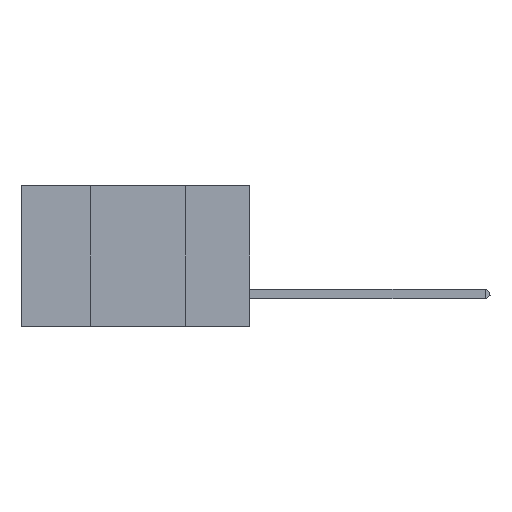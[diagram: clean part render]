
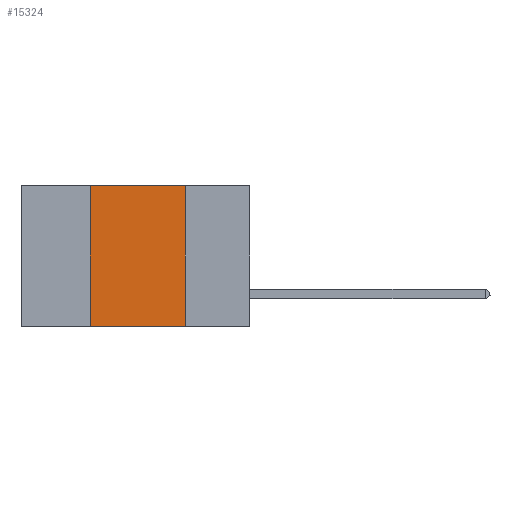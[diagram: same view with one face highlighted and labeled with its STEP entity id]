
A CAD part, left-side view. The second image highlights one B-rep face of the part: STEP entity #15324.
In plain terms, the highlighted planar face has unit normal (-1, 0, 0).
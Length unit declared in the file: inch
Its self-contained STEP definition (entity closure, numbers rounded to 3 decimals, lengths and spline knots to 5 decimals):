
#108 = LINE ( 'NONE', #15495, #8245 ) ;
#573 = CARTESIAN_POINT ( 'NONE',  ( 0., 0.17, -0.37 ) ) ;
#959 = EDGE_CURVE ( 'NONE', #5335, #7180, #17322, .T. ) ;
#1758 = AXIS2_PLACEMENT_3D ( 'NONE', #15825, #25925, #21804 ) ;
#2812 = EDGE_CURVE ( 'NONE', #5335, #7797, #108, .T. ) ;
#3399 = DIRECTION ( 'NONE',  ( 0., 0., 1. ) ) ;
#3773 = VERTEX_POINT ( 'NONE', #26687 ) ;
#4898 = CARTESIAN_POINT ( 'NONE',  ( 0., 0.6, -0.37 ) ) ;
#5335 = VERTEX_POINT ( 'NONE', #13394 ) ;
#6861 = DIRECTION ( 'NONE',  ( 0., -1., 0. ) ) ;
#7116 = LINE ( 'NONE', #11956, #24503 ) ;
#7180 = VERTEX_POINT ( 'NONE', #573 ) ;
#7212 = EDGE_CURVE ( 'NONE', #3773, #7180, #16054, .T. ) ;
#7395 = ORIENTED_EDGE ( 'NONE', *, *, #7212, .F. ) ;
#7797 = VERTEX_POINT ( 'NONE', #9765 ) ;
#8245 = VECTOR ( 'NONE', #3399, 39.37008 ) ;
#8473 = ORIENTED_EDGE ( 'NONE', *, *, #959, .T. ) ;
#9765 = CARTESIAN_POINT ( 'NONE',  ( 0., 0.42, 0. ) ) ;
#11023 = CARTESIAN_POINT ( 'NONE',  ( 0., 0.17, 0. ) ) ;
#11055 = EDGE_LOOP ( 'NONE', ( #7395, #13059, #12488, #8473 ) ) ;
#11956 = CARTESIAN_POINT ( 'NONE',  ( 0., 0.6, 0. ) ) ;
#12488 = ORIENTED_EDGE ( 'NONE', *, *, #2812, .F. ) ;
#13059 = ORIENTED_EDGE ( 'NONE', *, *, #24034, .F. ) ;
#13394 = CARTESIAN_POINT ( 'NONE',  ( 0., 0.42, -0.37 ) ) ;
#15324 = ADVANCED_FACE ( 'NONE', ( #18952 ), #23664, .F. ) ;
#15495 = CARTESIAN_POINT ( 'NONE',  ( 0., 0.42, 0. ) ) ;
#15825 = CARTESIAN_POINT ( 'NONE',  ( 0., 0.6, 0. ) ) ;
#16054 = LINE ( 'NONE', #11023, #20255 ) ;
#17322 = LINE ( 'NONE', #4898, #24730 ) ;
#18929 = DIRECTION ( 'NONE',  ( 0., 0., -1. ) ) ;
#18952 = FACE_OUTER_BOUND ( 'NONE', #11055, .T. ) ;
#20255 = VECTOR ( 'NONE', #18929, 39.37008 ) ;
#20399 = DIRECTION ( 'NONE',  ( 0., -1., 0. ) ) ;
#21804 = DIRECTION ( 'NONE',  ( 0., 0., -1. ) ) ;
#23664 = PLANE ( 'NONE',  #1758 ) ;
#24034 = EDGE_CURVE ( 'NONE', #7797, #3773, #7116, .T. ) ;
#24503 = VECTOR ( 'NONE', #20399, 39.37008 ) ;
#24730 = VECTOR ( 'NONE', #6861, 39.37008 ) ;
#25925 = DIRECTION ( 'NONE',  ( 1., 0., 0. ) ) ;
#26687 = CARTESIAN_POINT ( 'NONE',  ( 0., 0.17, 0. ) ) ;
